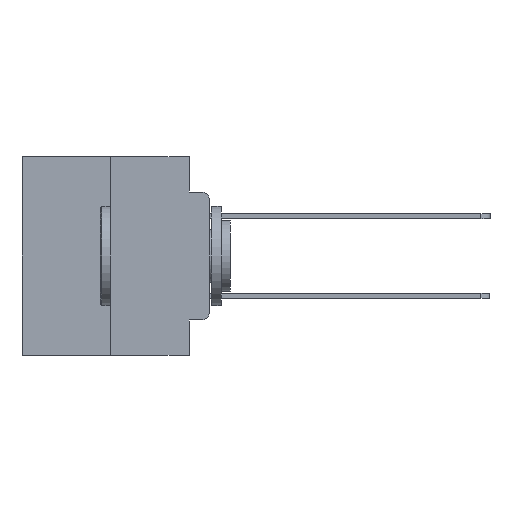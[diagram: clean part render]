
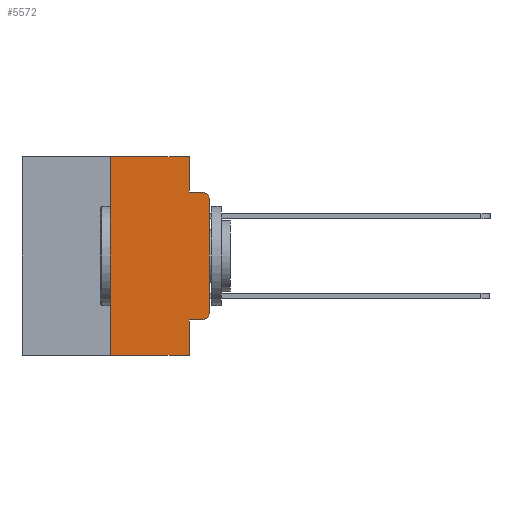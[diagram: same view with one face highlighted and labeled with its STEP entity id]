
A CAD part, left-side view. The second image highlights one B-rep face of the part: STEP entity #5572.
In plain terms, the highlighted planar face has unit normal (-1, 0, 0).
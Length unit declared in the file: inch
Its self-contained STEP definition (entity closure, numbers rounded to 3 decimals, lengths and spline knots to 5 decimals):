
#414 = CARTESIAN_POINT ( 'NONE',  ( 0., 0.051, -0.4115 ) ) ;
#477 = AXIS2_PLACEMENT_3D ( 'NONE', #12407, #27704, #14635 ) ;
#883 = VECTOR ( 'NONE', #21769, 39.37008 ) ;
#1013 = ORIENTED_EDGE ( 'NONE', *, *, #4337, .F. ) ;
#1863 = DIRECTION ( 'NONE',  ( 1., 0., 0. ) ) ;
#2307 = CARTESIAN_POINT ( 'NONE',  ( 0., 0.02, -0.0885 ) ) ;
#2698 = CARTESIAN_POINT ( 'NONE',  ( 0., 0.02, -0.3915 ) ) ;
#2710 = EDGE_LOOP ( 'NONE', ( #3523, #10249, #4947, #28423, #17527, #1013, #13056, #20253, #9927, #22315 ) ) ;
#3348 = VERTEX_POINT ( 'NONE', #16789 ) ;
#3523 = ORIENTED_EDGE ( 'NONE', *, *, #25899, .T. ) ;
#3998 = LINE ( 'NONE', #10876, #24809 ) ;
#4003 = CARTESIAN_POINT ( 'NONE',  ( 0., 0.051, -0.4115 ) ) ;
#4068 = CARTESIAN_POINT ( 'NONE',  ( 0., 0.051, -0.5 ) ) ;
#4337 = EDGE_CURVE ( 'NONE', #25156, #23744, #13718, .T. ) ;
#4947 = ORIENTED_EDGE ( 'NONE', *, *, #20723, .F. ) ;
#4976 = DIRECTION ( 'NONE',  ( 0., 0., -1. ) ) ;
#5153 = LINE ( 'NONE', #19738, #27933 ) ;
#5515 = AXIS2_PLACEMENT_3D ( 'NONE', #26212, #1863, #17530 ) ;
#5572 = ADVANCED_FACE ( 'NONE', ( #10891 ), #6233, .F. ) ;
#5612 = CARTESIAN_POINT ( 'NONE',  ( 0., 0.473, 0. ) ) ;
#6233 = PLANE ( 'NONE',  #5515 ) ;
#6335 = VECTOR ( 'NONE', #6598, 39.37008 ) ;
#6598 = DIRECTION ( 'NONE',  ( 0., 0., 1. ) ) ;
#6676 = CIRCLE ( 'NONE', #9385, 0.02 ) ;
#7004 = VERTEX_POINT ( 'NONE', #16466 ) ;
#7360 = LINE ( 'NONE', #5612, #24973 ) ;
#8337 = VECTOR ( 'NONE', #26941, 39.37008 ) ;
#8347 = VERTEX_POINT ( 'NONE', #20861 ) ;
#8385 = DIRECTION ( 'NONE',  ( 0., 0., -1. ) ) ;
#9385 = AXIS2_PLACEMENT_3D ( 'NONE', #2698, #18323, #4976 ) ;
#9927 = ORIENTED_EDGE ( 'NONE', *, *, #24378, .T. ) ;
#10249 = ORIENTED_EDGE ( 'NONE', *, *, #21650, .T. ) ;
#10876 = CARTESIAN_POINT ( 'NONE',  ( 0., 0.051, 0. ) ) ;
#10891 = FACE_OUTER_BOUND ( 'NONE', #2710, .T. ) ;
#11886 = VERTEX_POINT ( 'NONE', #4068 ) ;
#11890 = EDGE_CURVE ( 'NONE', #26546, #3348, #3998, .T. ) ;
#12407 = CARTESIAN_POINT ( 'NONE',  ( 0., 0.02, -0.1085 ) ) ;
#13056 = ORIENTED_EDGE ( 'NONE', *, *, #18685, .T. ) ;
#13718 = LINE ( 'NONE', #26472, #6335 ) ;
#13990 = VERTEX_POINT ( 'NONE', #414 ) ;
#14032 = LINE ( 'NONE', #17796, #17793 ) ;
#14397 = VECTOR ( 'NONE', #8385, 39.37008 ) ;
#14635 = DIRECTION ( 'NONE',  ( 0., 0., -1. ) ) ;
#14742 = CARTESIAN_POINT ( 'NONE',  ( 0., 0.25, 0. ) ) ;
#14958 = LINE ( 'NONE', #24766, #8337 ) ;
#15000 = CARTESIAN_POINT ( 'NONE',  ( 0., 0.051, 0. ) ) ;
#15215 = EDGE_CURVE ( 'NONE', #13990, #11886, #20199, .T. ) ;
#15360 = DIRECTION ( 'NONE',  ( 0., -1., 0. ) ) ;
#15425 = VERTEX_POINT ( 'NONE', #2307 ) ;
#15519 = EDGE_CURVE ( 'NONE', #8347, #7004, #6676, .T. ) ;
#15632 = CARTESIAN_POINT ( 'NONE',  ( 0., 0.25, -0.5 ) ) ;
#16466 = CARTESIAN_POINT ( 'NONE',  ( 0., 0., -0.3915 ) ) ;
#16789 = CARTESIAN_POINT ( 'NONE',  ( 0., 0.051, -0.0885 ) ) ;
#17527 = ORIENTED_EDGE ( 'NONE', *, *, #23707, .F. ) ;
#17530 = DIRECTION ( 'NONE',  ( 0., 0., -1. ) ) ;
#17793 = VECTOR ( 'NONE', #19985, 39.37008 ) ;
#17796 = CARTESIAN_POINT ( 'NONE',  ( 0., 0.473, -0.5 ) ) ;
#18323 = DIRECTION ( 'NONE',  ( -1., 0., 0. ) ) ;
#18685 = EDGE_CURVE ( 'NONE', #25156, #11886, #14032, .T. ) ;
#18957 = DIRECTION ( 'NONE',  ( 0., -1., 0. ) ) ;
#19013 = VERTEX_POINT ( 'NONE', #21103 ) ;
#19738 = CARTESIAN_POINT ( 'NONE',  ( 0., 0.051, -0.0885 ) ) ;
#19985 = DIRECTION ( 'NONE',  ( 0., -1., 0. ) ) ;
#20199 = LINE ( 'NONE', #15000, #14397 ) ;
#20253 = ORIENTED_EDGE ( 'NONE', *, *, #15215, .F. ) ;
#20723 = EDGE_CURVE ( 'NONE', #3348, #15425, #5153, .T. ) ;
#20861 = CARTESIAN_POINT ( 'NONE',  ( 0., 0.02, -0.4115 ) ) ;
#20948 = CARTESIAN_POINT ( 'NONE',  ( 0., 0.051, 0. ) ) ;
#21103 = CARTESIAN_POINT ( 'NONE',  ( 0., 0., -0.1085 ) ) ;
#21650 = EDGE_CURVE ( 'NONE', #19013, #15425, #22096, .T. ) ;
#21769 = DIRECTION ( 'NONE',  ( 0., -1., 0. ) ) ;
#22096 = CIRCLE ( 'NONE', #477, 0.02 ) ;
#22315 = ORIENTED_EDGE ( 'NONE', *, *, #15519, .T. ) ;
#23707 = EDGE_CURVE ( 'NONE', #23744, #26546, #7360, .T. ) ;
#23744 = VERTEX_POINT ( 'NONE', #14742 ) ;
#24378 = EDGE_CURVE ( 'NONE', #13990, #8347, #24584, .T. ) ;
#24584 = LINE ( 'NONE', #4003, #883 ) ;
#24766 = CARTESIAN_POINT ( 'NONE',  ( 0., 0., 0. ) ) ;
#24809 = VECTOR ( 'NONE', #26230, 39.37008 ) ;
#24973 = VECTOR ( 'NONE', #18957, 39.37008 ) ;
#25156 = VERTEX_POINT ( 'NONE', #15632 ) ;
#25899 = EDGE_CURVE ( 'NONE', #7004, #19013, #14958, .T. ) ;
#26212 = CARTESIAN_POINT ( 'NONE',  ( 0., 0.473, 0. ) ) ;
#26230 = DIRECTION ( 'NONE',  ( 0., 0., -1. ) ) ;
#26472 = CARTESIAN_POINT ( 'NONE',  ( 0., 0.25, 0. ) ) ;
#26546 = VERTEX_POINT ( 'NONE', #20948 ) ;
#26941 = DIRECTION ( 'NONE',  ( 0., 0., 1. ) ) ;
#27704 = DIRECTION ( 'NONE',  ( -1., 0., 0. ) ) ;
#27933 = VECTOR ( 'NONE', #15360, 39.37008 ) ;
#28423 = ORIENTED_EDGE ( 'NONE', *, *, #11890, .F. ) ;
